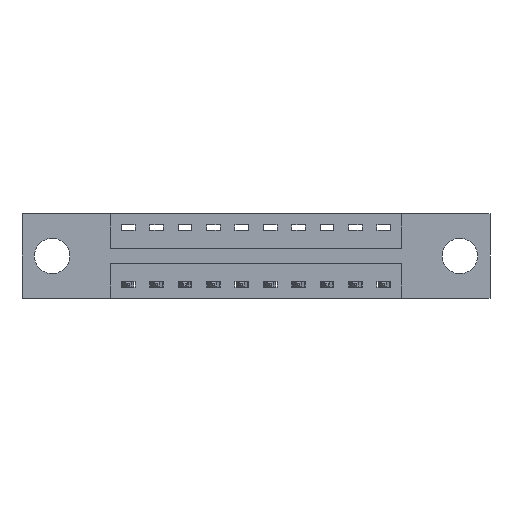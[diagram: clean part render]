
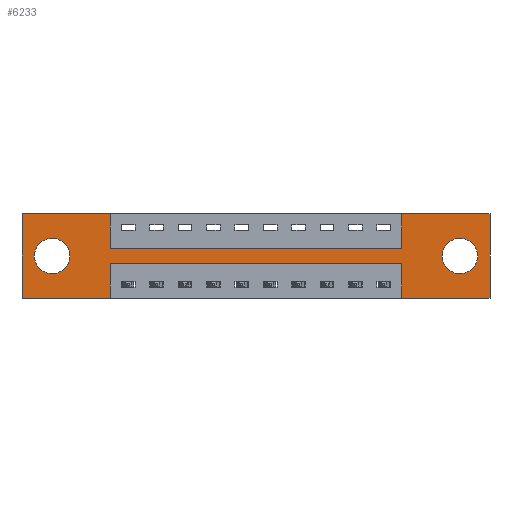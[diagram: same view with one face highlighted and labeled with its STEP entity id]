
A CAD part, front view. The second image highlights one B-rep face of the part: STEP entity #6233.
In plain terms, the highlighted planar face has unit normal (0, -1, 0).
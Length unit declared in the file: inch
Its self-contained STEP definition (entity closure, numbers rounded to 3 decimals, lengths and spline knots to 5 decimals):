
#48 = VECTOR ( 'NONE', #1620, 39.37008 ) ;
#58 = EDGE_CURVE ( 'NONE', #948, #6850, #2775, .T. ) ;
#235 = LINE ( 'NONE', #4365, #559 ) ;
#362 = FACE_OUTER_BOUND ( 'NONE', #5527, .T. ) ;
#380 = ORIENTED_EDGE ( 'NONE', *, *, #8341, .F. ) ;
#395 = DIRECTION ( 'NONE',  ( -1., 0., 0. ) ) ;
#484 = CARTESIAN_POINT ( 'NONE',  ( 2.06, 0., 0. ) ) ;
#559 = VECTOR ( 'NONE', #395, 39.37008 ) ;
#631 = VERTEX_POINT ( 'NONE', #2746 ) ;
#663 = CARTESIAN_POINT ( 'NONE',  ( 2.06, 0., -0.37 ) ) ;
#692 = VECTOR ( 'NONE', #7422, 39.37008 ) ;
#755 = ORIENTED_EDGE ( 'NONE', *, *, #9558, .F. ) ;
#948 = VERTEX_POINT ( 'NONE', #5561 ) ;
#959 = DIRECTION ( 'NONE',  ( 0., 1., 0. ) ) ;
#976 = ORIENTED_EDGE ( 'NONE', *, *, #7220, .F. ) ;
#1064 = VECTOR ( 'NONE', #4754, 39.37008 ) ;
#1160 = VECTOR ( 'NONE', #7548, 39.37008 ) ;
#1278 = VECTOR ( 'NONE', #10926, 39.37008 ) ;
#1290 = LINE ( 'NONE', #10468, #8493 ) ;
#1342 = CIRCLE ( 'NONE', #7575, 0.078 ) ;
#1361 = AXIS2_PLACEMENT_3D ( 'NONE', #3260, #2236, #5636 ) ;
#1534 = CARTESIAN_POINT ( 'NONE',  ( 0.1325, 0., -0.185 ) ) ;
#1538 = VERTEX_POINT ( 'NONE', #4800 ) ;
#1620 = DIRECTION ( 'NONE',  ( 0., 0., 1. ) ) ;
#2011 = VERTEX_POINT ( 'NONE', #4679 ) ;
#2191 = VERTEX_POINT ( 'NONE', #7279 ) ;
#2215 = CIRCLE ( 'NONE', #2936, 0.078 ) ;
#2236 = DIRECTION ( 'NONE',  ( 0., 1., 0. ) ) ;
#2327 = DIRECTION ( 'NONE',  ( 0., 0., 1. ) ) ;
#2376 = DIRECTION ( 'NONE',  ( 0., 1., 0. ) ) ;
#2426 = VERTEX_POINT ( 'NONE', #8349 ) ;
#2445 = EDGE_CURVE ( 'NONE', #2426, #3561, #7497, .T. ) ;
#2449 = VERTEX_POINT ( 'NONE', #663 ) ;
#2495 = CARTESIAN_POINT ( 'NONE',  ( 0.1325, 0., -0.185 ) ) ;
#2716 = DIRECTION ( 'NONE',  ( 0., -1., 0. ) ) ;
#2746 = CARTESIAN_POINT ( 'NONE',  ( 1.6725, 0., -0.15 ) ) ;
#2775 = CIRCLE ( 'NONE', #1361, 0.078 ) ;
#2884 = FACE_BOUND ( 'NONE', #9319, .T. ) ;
#2936 = AXIS2_PLACEMENT_3D ( 'NONE', #2495, #2376, #5888 ) ;
#2946 = ORIENTED_EDGE ( 'NONE', *, *, #8897, .F. ) ;
#2978 = VERTEX_POINT ( 'NONE', #10966 ) ;
#3058 = VERTEX_POINT ( 'NONE', #6980 ) ;
#3260 = CARTESIAN_POINT ( 'NONE',  ( 1.9275, 0., -0.185 ) ) ;
#3262 = VECTOR ( 'NONE', #8044, 39.37008 ) ;
#3293 = ORIENTED_EDGE ( 'NONE', *, *, #8687, .F. ) ;
#3378 = VERTEX_POINT ( 'NONE', #6675 ) ;
#3527 = ORIENTED_EDGE ( 'NONE', *, *, #10027, .T. ) ;
#3561 = VERTEX_POINT ( 'NONE', #4516 ) ;
#3592 = LINE ( 'NONE', #484, #4963 ) ;
#3615 = PLANE ( 'NONE',  #7269 ) ;
#3626 = CIRCLE ( 'NONE', #4159, 0.078 ) ;
#3637 = CARTESIAN_POINT ( 'NONE',  ( 0., 0., 0. ) ) ;
#3879 = LINE ( 'NONE', #6278, #9114 ) ;
#3985 = CARTESIAN_POINT ( 'NONE',  ( 0.3875, 0., -0.37 ) ) ;
#4131 = CARTESIAN_POINT ( 'NONE',  ( 0.1325, 0., -0.263 ) ) ;
#4159 = AXIS2_PLACEMENT_3D ( 'NONE', #1534, #8095, #2327 ) ;
#4325 = LINE ( 'NONE', #10014, #1278 ) ;
#4348 = ORIENTED_EDGE ( 'NONE', *, *, #10237, .F. ) ;
#4349 = DIRECTION ( 'NONE',  ( 0., 0., -1. ) ) ;
#4365 = CARTESIAN_POINT ( 'NONE',  ( 0.3875, 0., -0.22 ) ) ;
#4401 = ORIENTED_EDGE ( 'NONE', *, *, #9905, .F. ) ;
#4516 = CARTESIAN_POINT ( 'NONE',  ( 0.3875, 0., -0.37 ) ) ;
#4679 = CARTESIAN_POINT ( 'NONE',  ( 2.06, 0., 0. ) ) ;
#4709 = EDGE_CURVE ( 'NONE', #6850, #948, #1342, .T. ) ;
#4754 = DIRECTION ( 'NONE',  ( 0., 0., -1. ) ) ;
#4800 = CARTESIAN_POINT ( 'NONE',  ( 0.3875, 0., -0.15 ) ) ;
#4963 = VECTOR ( 'NONE', #7897, 39.37008 ) ;
#5056 = CARTESIAN_POINT ( 'NONE',  ( 1.9275, 0., -0.185 ) ) ;
#5062 = CARTESIAN_POINT ( 'NONE',  ( 1.6725, 0., -0.37 ) ) ;
#5102 = LINE ( 'NONE', #8433, #8741 ) ;
#5210 = CARTESIAN_POINT ( 'NONE',  ( 0., 0., 0. ) ) ;
#5527 = EDGE_LOOP ( 'NONE', ( #8352, #9291, #755, #3293, #976, #8069, #4348, #10252, #6702, #2946, #4401, #380 ) ) ;
#5561 = CARTESIAN_POINT ( 'NONE',  ( 1.9275, 0., -0.107 ) ) ;
#5636 = DIRECTION ( 'NONE',  ( 0., 0., -1. ) ) ;
#5888 = DIRECTION ( 'NONE',  ( 0., 0., 1. ) ) ;
#6068 = EDGE_CURVE ( 'NONE', #1538, #631, #5102, .T. ) ;
#6130 = EDGE_LOOP ( 'NONE', ( #9729, #3527 ) ) ;
#6233 = ADVANCED_FACE ( 'NONE', ( #2884, #7176, #362 ), #3615, .T. ) ;
#6278 = CARTESIAN_POINT ( 'NONE',  ( 1.6725, 0., 0. ) ) ;
#6523 = ORIENTED_EDGE ( 'NONE', *, *, #58, .T. ) ;
#6675 = CARTESIAN_POINT ( 'NONE',  ( 1.6725, 0., 0. ) ) ;
#6702 = ORIENTED_EDGE ( 'NONE', *, *, #7609, .F. ) ;
#6756 = LINE ( 'NONE', #9351, #1160 ) ;
#6850 = VERTEX_POINT ( 'NONE', #10218 ) ;
#6980 = CARTESIAN_POINT ( 'NONE',  ( 1.6725, 0., -0.22 ) ) ;
#7176 = FACE_BOUND ( 'NONE', #6130, .T. ) ;
#7220 = EDGE_CURVE ( 'NONE', #2011, #2449, #3592, .T. ) ;
#7269 = AXIS2_PLACEMENT_3D ( 'NONE', #9673, #2716, #9723 ) ;
#7279 = CARTESIAN_POINT ( 'NONE',  ( 0.1325, 0., -0.107 ) ) ;
#7309 = DIRECTION ( 'NONE',  ( 0., 0., 1. ) ) ;
#7372 = VERTEX_POINT ( 'NONE', #4131 ) ;
#7421 = LINE ( 'NONE', #5062, #48 ) ;
#7422 = DIRECTION ( 'NONE',  ( 1., 0., 0. ) ) ;
#7451 = VERTEX_POINT ( 'NONE', #7755 ) ;
#7478 = ORIENTED_EDGE ( 'NONE', *, *, #4709, .T. ) ;
#7497 = LINE ( 'NONE', #3985, #1064 ) ;
#7548 = DIRECTION ( 'NONE',  ( -1., 0., 0. ) ) ;
#7575 = AXIS2_PLACEMENT_3D ( 'NONE', #5056, #959, #4349 ) ;
#7609 = EDGE_CURVE ( 'NONE', #9103, #1538, #9764, .T. ) ;
#7722 = EDGE_CURVE ( 'NONE', #2191, #7372, #3626, .T. ) ;
#7755 = CARTESIAN_POINT ( 'NONE',  ( 1.6725, 0., -0.37 ) ) ;
#7897 = DIRECTION ( 'NONE',  ( 0., 0., -1. ) ) ;
#7922 = CARTESIAN_POINT ( 'NONE',  ( 0.3875, 0., 0. ) ) ;
#8044 = DIRECTION ( 'NONE',  ( 0., 0., -1. ) ) ;
#8069 = ORIENTED_EDGE ( 'NONE', *, *, #10890, .F. ) ;
#8095 = DIRECTION ( 'NONE',  ( 0., 1., 0. ) ) ;
#8341 = EDGE_CURVE ( 'NONE', #3561, #2978, #4325, .T. ) ;
#8349 = CARTESIAN_POINT ( 'NONE',  ( 0.3875, 0., -0.22 ) ) ;
#8352 = ORIENTED_EDGE ( 'NONE', *, *, #2445, .F. ) ;
#8433 = CARTESIAN_POINT ( 'NONE',  ( 0.3875, 0., -0.15 ) ) ;
#8493 = VECTOR ( 'NONE', #7309, 39.37008 ) ;
#8645 = CARTESIAN_POINT ( 'NONE',  ( 0.3875, 0., 0. ) ) ;
#8669 = LINE ( 'NONE', #3637, #10402 ) ;
#8687 = EDGE_CURVE ( 'NONE', #2449, #7451, #6756, .T. ) ;
#8741 = VECTOR ( 'NONE', #10187, 39.37008 ) ;
#8897 = EDGE_CURVE ( 'NONE', #9109, #9103, #8669, .T. ) ;
#9103 = VERTEX_POINT ( 'NONE', #8645 ) ;
#9109 = VERTEX_POINT ( 'NONE', #5210 ) ;
#9114 = VECTOR ( 'NONE', #9819, 39.37008 ) ;
#9291 = ORIENTED_EDGE ( 'NONE', *, *, #10497, .F. ) ;
#9298 = LINE ( 'NONE', #10148, #692 ) ;
#9319 = EDGE_LOOP ( 'NONE', ( #6523, #7478 ) ) ;
#9351 = CARTESIAN_POINT ( 'NONE',  ( 0., 0., -0.37 ) ) ;
#9558 = EDGE_CURVE ( 'NONE', #7451, #3058, #7421, .T. ) ;
#9673 = CARTESIAN_POINT ( 'NONE',  ( 0., 0., -0.37 ) ) ;
#9723 = DIRECTION ( 'NONE',  ( 0., 0., -1. ) ) ;
#9729 = ORIENTED_EDGE ( 'NONE', *, *, #7722, .T. ) ;
#9764 = LINE ( 'NONE', #7922, #3262 ) ;
#9819 = DIRECTION ( 'NONE',  ( 0., 0., 1. ) ) ;
#9905 = EDGE_CURVE ( 'NONE', #2978, #9109, #1290, .T. ) ;
#10014 = CARTESIAN_POINT ( 'NONE',  ( 0., 0., -0.37 ) ) ;
#10027 = EDGE_CURVE ( 'NONE', #7372, #2191, #2215, .T. ) ;
#10148 = CARTESIAN_POINT ( 'NONE',  ( 0., 0., 0. ) ) ;
#10187 = DIRECTION ( 'NONE',  ( 1., 0., 0. ) ) ;
#10218 = CARTESIAN_POINT ( 'NONE',  ( 1.9275, 0., -0.263 ) ) ;
#10237 = EDGE_CURVE ( 'NONE', #631, #3378, #3879, .T. ) ;
#10252 = ORIENTED_EDGE ( 'NONE', *, *, #6068, .F. ) ;
#10402 = VECTOR ( 'NONE', #10422, 39.37008 ) ;
#10422 = DIRECTION ( 'NONE',  ( 1., 0., 0. ) ) ;
#10468 = CARTESIAN_POINT ( 'NONE',  ( 0., 0., 0. ) ) ;
#10497 = EDGE_CURVE ( 'NONE', #3058, #2426, #235, .T. ) ;
#10890 = EDGE_CURVE ( 'NONE', #3378, #2011, #9298, .T. ) ;
#10926 = DIRECTION ( 'NONE',  ( -1., 0., 0. ) ) ;
#10966 = CARTESIAN_POINT ( 'NONE',  ( 0., 0., -0.37 ) ) ;
